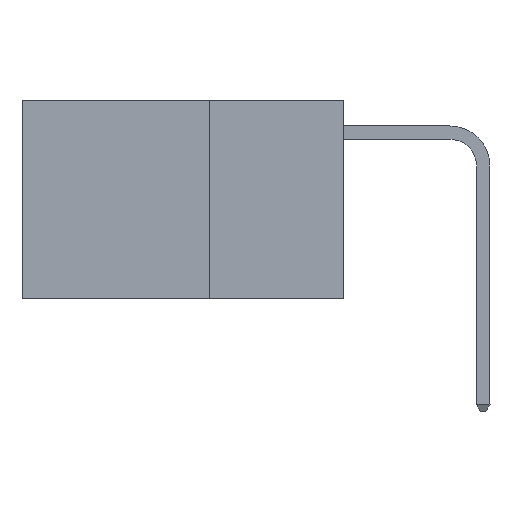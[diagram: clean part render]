
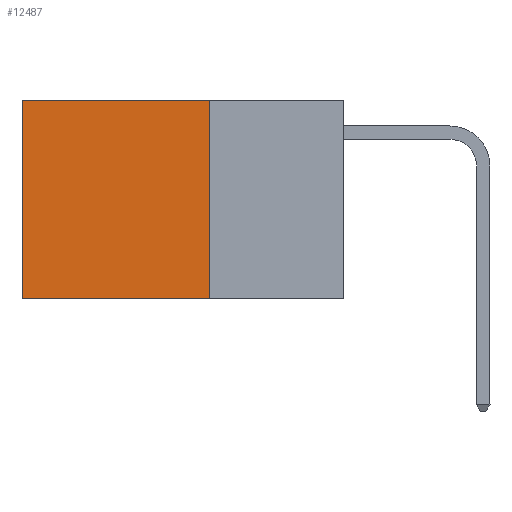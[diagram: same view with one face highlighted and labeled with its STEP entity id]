
A CAD part, left-side view. The second image highlights one B-rep face of the part: STEP entity #12487.
In plain terms, the highlighted planar face has unit normal (-1, 0, 0).
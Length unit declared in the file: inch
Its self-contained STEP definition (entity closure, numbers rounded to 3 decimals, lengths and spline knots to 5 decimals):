
#335 = ORIENTED_EDGE ( 'NONE', *, *, #3699, .T. ) ;
#682 = FACE_OUTER_BOUND ( 'NONE', #1208, .T. ) ;
#755 = LINE ( 'NONE', #2148, #871 ) ;
#871 = VECTOR ( 'NONE', #1668, 39.37008 ) ;
#1028 = DIRECTION ( 'NONE',  ( 1., 0., 0. ) ) ;
#1126 = VERTEX_POINT ( 'NONE', #5850 ) ;
#1206 = LINE ( 'NONE', #3918, #1456 ) ;
#1208 = EDGE_LOOP ( 'NONE', ( #335, #10694, #5302, #8776 ) ) ;
#1222 = AXIS2_PLACEMENT_3D ( 'NONE', #12064, #1028, #8310 ) ;
#1279 = VERTEX_POINT ( 'NONE', #8061 ) ;
#1456 = VECTOR ( 'NONE', #6544, 39.37008 ) ;
#1509 = LINE ( 'NONE', #4651, #1703 ) ;
#1668 = DIRECTION ( 'NONE',  ( 0., 0., -1. ) ) ;
#1703 = VECTOR ( 'NONE', #4641, 39.37008 ) ;
#2148 = CARTESIAN_POINT ( 'NONE',  ( 0.2625, 0.25, 0. ) ) ;
#2461 = EDGE_CURVE ( 'NONE', #1126, #7314, #1206, .T. ) ;
#3699 = EDGE_CURVE ( 'NONE', #1279, #7314, #6992, .T. ) ;
#3918 = CARTESIAN_POINT ( 'NONE',  ( 0.2625, 0.25, -0.37 ) ) ;
#4499 = CARTESIAN_POINT ( 'NONE',  ( 0.2625, 0.6, -0.37 ) ) ;
#4641 = DIRECTION ( 'NONE',  ( 0., 1., 0. ) ) ;
#4651 = CARTESIAN_POINT ( 'NONE',  ( 0.2625, 0.25, 0. ) ) ;
#5302 = ORIENTED_EDGE ( 'NONE', *, *, #9797, .F. ) ;
#5850 = CARTESIAN_POINT ( 'NONE',  ( 0.2625, 0.25, -0.37 ) ) ;
#6544 = DIRECTION ( 'NONE',  ( 0., 1., 0. ) ) ;
#6981 = VECTOR ( 'NONE', #9656, 39.37008 ) ;
#6992 = LINE ( 'NONE', #9772, #6981 ) ;
#7314 = VERTEX_POINT ( 'NONE', #4499 ) ;
#7747 = CARTESIAN_POINT ( 'NONE',  ( 0.2625, 0.25, 0. ) ) ;
#8061 = CARTESIAN_POINT ( 'NONE',  ( 0.2625, 0.6, 0. ) ) ;
#8310 = DIRECTION ( 'NONE',  ( 0., 0., -1. ) ) ;
#8776 = ORIENTED_EDGE ( 'NONE', *, *, #11078, .T. ) ;
#9656 = DIRECTION ( 'NONE',  ( 0., 0., -1. ) ) ;
#9772 = CARTESIAN_POINT ( 'NONE',  ( 0.2625, 0.6, 0. ) ) ;
#9797 = EDGE_CURVE ( 'NONE', #10682, #1126, #755, .T. ) ;
#10682 = VERTEX_POINT ( 'NONE', #7747 ) ;
#10694 = ORIENTED_EDGE ( 'NONE', *, *, #2461, .F. ) ;
#11078 = EDGE_CURVE ( 'NONE', #10682, #1279, #1509, .T. ) ;
#12064 = CARTESIAN_POINT ( 'NONE',  ( 0.2625, 0.25, 0. ) ) ;
#12487 = ADVANCED_FACE ( 'NONE', ( #682 ), #12863, .F. ) ;
#12863 = PLANE ( 'NONE',  #1222 ) ;
